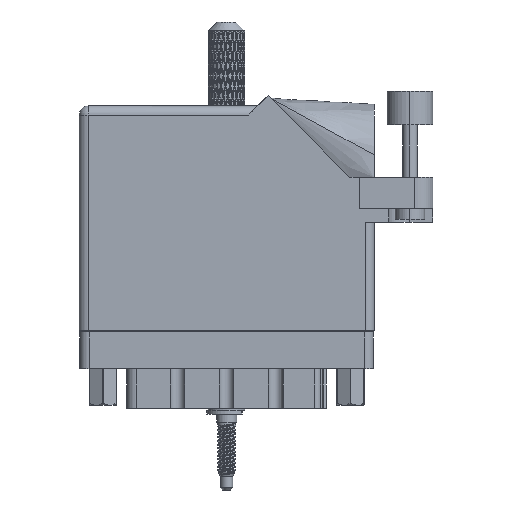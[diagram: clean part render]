
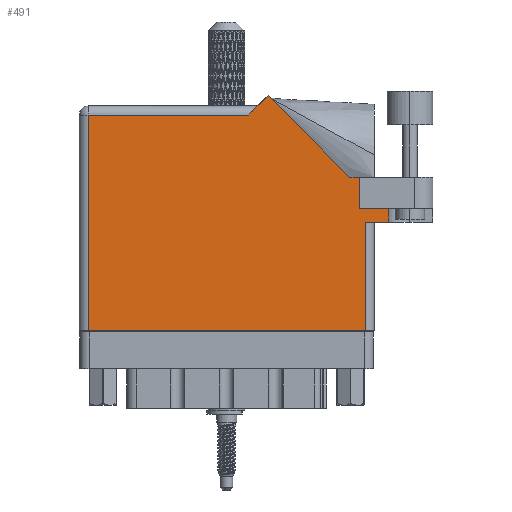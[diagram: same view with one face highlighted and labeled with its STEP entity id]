
A CAD part, front view. The second image highlights one B-rep face of the part: STEP entity #491.
In plain terms, the highlighted face is planar.
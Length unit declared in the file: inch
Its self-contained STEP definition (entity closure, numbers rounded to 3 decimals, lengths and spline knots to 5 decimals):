
#400 = ORIENTED_EDGE ( 'NONE', *, *, #1383, .T. ) ;
#491 = ADVANCED_FACE ( 'NONE', ( #113751 ), #7438, .F. ) ;
#534 = CARTESIAN_POINT ( 'NONE',  ( 1.28771, 1.60071, 0. ) ) ;
#1239 = DIRECTION ( 'NONE',  ( -1., 0., 0. ) ) ;
#1383 = EDGE_CURVE ( 'NONE', #14926, #71492, #99734, .T. ) ;
#1957 = CARTESIAN_POINT ( 'NONE',  ( 2.1115, 1.16177, 0. ) ) ;
#2376 = EDGE_CURVE ( 'NONE', #78293, #14926, #14545, .T. ) ;
#4260 = DIRECTION ( 'NONE',  ( -0.707, 0.707, 0. ) ) ;
#4875 = CARTESIAN_POINT ( 'NONE',  ( 1.948, 0.737, 0. ) ) ;
#5803 = CARTESIAN_POINT ( 'NONE',  ( 0., 0., 0. ) ) ;
#6280 = DIRECTION ( 'NONE',  ( -1., 0., 0. ) ) ;
#7240 = VERTEX_POINT ( 'NONE', #8435 ) ;
#7438 = PLANE ( 'NONE',  #97982 ) ;
#7936 = ORIENTED_EDGE ( 'NONE', *, *, #35470, .T. ) ;
#8435 = CARTESIAN_POINT ( 'NONE',  ( 2.1115, 0.831, 0. ) ) ;
#9878 = ORIENTED_EDGE ( 'NONE', *, *, #10628, .F. ) ;
#10516 = DIRECTION ( 'NONE',  ( 0., -1., 0. ) ) ;
#10628 = EDGE_CURVE ( 'NONE', #7240, #71492, #82411, .T. ) ;
#11083 = CARTESIAN_POINT ( 'NONE',  ( 2.1115, 0.737, 0. ) ) ;
#11648 = DIRECTION ( 'NONE',  ( 1., 0., 0. ) ) ;
#12313 = LINE ( 'NONE', #5803, #69215 ) ;
#13638 = LINE ( 'NONE', #111722, #85238 ) ;
#14545 = LINE ( 'NONE', #15700, #28859 ) ;
#14926 = VERTEX_POINT ( 'NONE', #4875 ) ;
#15700 = CARTESIAN_POINT ( 'NONE',  ( 1.948, 0.737, 0. ) ) ;
#18199 = CARTESIAN_POINT ( 'NONE',  ( 1.91, 1.044, 0. ) ) ;
#20411 = ORIENTED_EDGE ( 'NONE', *, *, #103364, .F. ) ;
#22264 = DIRECTION ( 'NONE',  ( 1., 0., 0. ) ) ;
#22705 = CARTESIAN_POINT ( 'NONE',  ( 1.948, 0., 0. ) ) ;
#28859 = VECTOR ( 'NONE', #103789, 39.37008 ) ;
#29074 = ORIENTED_EDGE ( 'NONE', *, *, #71429, .T. ) ;
#29904 = LINE ( 'NONE', #109743, #41256 ) ;
#30584 = VERTEX_POINT ( 'NONE', #86433 ) ;
#30913 = VECTOR ( 'NONE', #105643, 39.37008 ) ;
#31846 = VECTOR ( 'NONE', #65385, 39.37008 ) ;
#35470 = EDGE_CURVE ( 'NONE', #81924, #60542, #54098, .T. ) ;
#35644 = VECTOR ( 'NONE', #1239, 39.37008 ) ;
#38151 = ORIENTED_EDGE ( 'NONE', *, *, #38943, .T. ) ;
#38943 = EDGE_CURVE ( 'NONE', #60542, #75135, #29904, .T. ) ;
#39026 = VECTOR ( 'NONE', #63726, 39.37008 ) ;
#41166 = CARTESIAN_POINT ( 'NONE',  ( 1.155, 1.468, 0. ) ) ;
#41256 = VECTOR ( 'NONE', #10516, 39.37008 ) ;
#42968 = VECTOR ( 'NONE', #62633, 39.37008 ) ;
#44360 = CARTESIAN_POINT ( 'NONE',  ( 1.91, 0.831, 0. ) ) ;
#45014 = LINE ( 'NONE', #89058, #42968 ) ;
#45610 = ORIENTED_EDGE ( 'NONE', *, *, #53101, .T. ) ;
#53024 = EDGE_LOOP ( 'NONE', ( #107733, #112781, #400, #9878, #20411, #97322, #29074, #45610, #67586, #7936, #38151 ) ) ;
#53041 = CARTESIAN_POINT ( 'NONE',  ( 1.217, 1.53, 0. ) ) ;
#53101 = EDGE_CURVE ( 'NONE', #67366, #111370, #13638, .T. ) ;
#54098 = LINE ( 'NONE', #100466, #35644 ) ;
#60542 = VERTEX_POINT ( 'NONE', #61129 ) ;
#61129 = CARTESIAN_POINT ( 'NONE',  ( 0.062, 1.468, 0. ) ) ;
#62633 = DIRECTION ( 'NONE',  ( 0., 1., 0. ) ) ;
#63726 = DIRECTION ( 'NONE',  ( 1., 0., 0. ) ) ;
#65385 = DIRECTION ( 'NONE',  ( 0., -1., 0. ) ) ;
#67366 = VERTEX_POINT ( 'NONE', #75715 ) ;
#67586 = ORIENTED_EDGE ( 'NONE', *, *, #86386, .T. ) ;
#69215 = VECTOR ( 'NONE', #22264, 39.37008 ) ;
#71429 = EDGE_CURVE ( 'NONE', #106253, #67366, #78112, .T. ) ;
#71492 = VERTEX_POINT ( 'NONE', #11083 ) ;
#72545 = LINE ( 'NONE', #44360, #39026 ) ;
#75135 = VERTEX_POINT ( 'NONE', #94951 ) ;
#75715 = CARTESIAN_POINT ( 'NONE',  ( 1.84442, 1.044, 0. ) ) ;
#77764 = DIRECTION ( 'NONE',  ( -0.707, -0.707, 0. ) ) ;
#78112 = LINE ( 'NONE', #79822, #30913 ) ;
#78293 = VERTEX_POINT ( 'NONE', #22705 ) ;
#79822 = CARTESIAN_POINT ( 'NONE',  ( 2.41, 1.044, 0. ) ) ;
#81924 = VERTEX_POINT ( 'NONE', #41166 ) ;
#82411 = LINE ( 'NONE', #1957, #31846 ) ;
#85238 = VECTOR ( 'NONE', #4260, 39.37008 ) ;
#86173 = DIRECTION ( 'NONE',  ( 0., 0., -1. ) ) ;
#86386 = EDGE_CURVE ( 'NONE', #111370, #81924, #105876, .T. ) ;
#86433 = CARTESIAN_POINT ( 'NONE',  ( 1.91, 0.831, 0. ) ) ;
#89058 = CARTESIAN_POINT ( 'NONE',  ( 1.91, 0.831, 0. ) ) ;
#92272 = VECTOR ( 'NONE', #77764, 39.37008 ) ;
#94951 = CARTESIAN_POINT ( 'NONE',  ( 0.062, 0., 0. ) ) ;
#97322 = ORIENTED_EDGE ( 'NONE', *, *, #110172, .T. ) ;
#97982 = AXIS2_PLACEMENT_3D ( 'NONE', #114887, #86173, #6280 ) ;
#99734 = LINE ( 'NONE', #109104, #109376 ) ;
#100466 = CARTESIAN_POINT ( 'NONE',  ( 0., 1.468, 0. ) ) ;
#103364 = EDGE_CURVE ( 'NONE', #30584, #7240, #72545, .T. ) ;
#103789 = DIRECTION ( 'NONE',  ( 0., 1., 0. ) ) ;
#105530 = EDGE_CURVE ( 'NONE', #75135, #78293, #12313, .T. ) ;
#105643 = DIRECTION ( 'NONE',  ( -1., 0., 0. ) ) ;
#105876 = LINE ( 'NONE', #53041, #92272 ) ;
#106253 = VERTEX_POINT ( 'NONE', #18199 ) ;
#107733 = ORIENTED_EDGE ( 'NONE', *, *, #105530, .T. ) ;
#109104 = CARTESIAN_POINT ( 'NONE',  ( 2.01, 0.737, 0. ) ) ;
#109376 = VECTOR ( 'NONE', #11648, 39.37008 ) ;
#109743 = CARTESIAN_POINT ( 'NONE',  ( 0.062, 0., 0. ) ) ;
#110172 = EDGE_CURVE ( 'NONE', #30584, #106253, #45014, .T. ) ;
#111370 = VERTEX_POINT ( 'NONE', #534 ) ;
#111722 = CARTESIAN_POINT ( 'NONE',  ( 1.84442, 1.044, 0. ) ) ;
#112781 = ORIENTED_EDGE ( 'NONE', *, *, #2376, .T. ) ;
#113751 = FACE_OUTER_BOUND ( 'NONE', #53024, .T. ) ;
#114887 = CARTESIAN_POINT ( 'NONE',  ( 0., 1.53, 0. ) ) ;
